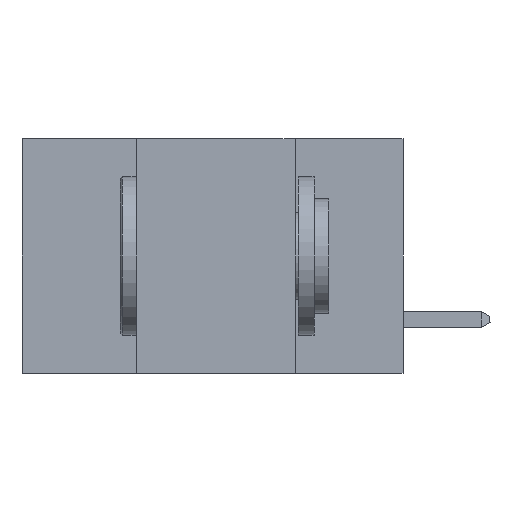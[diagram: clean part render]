
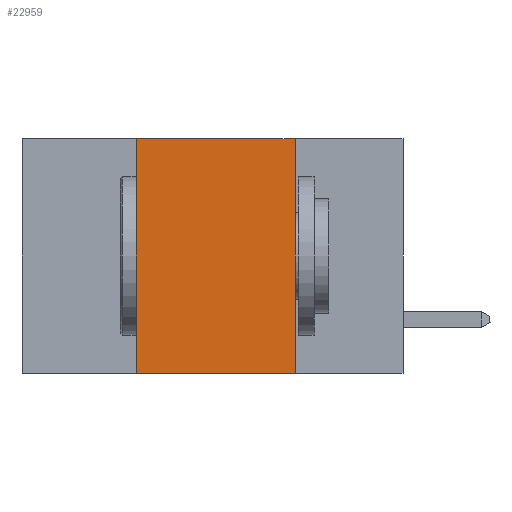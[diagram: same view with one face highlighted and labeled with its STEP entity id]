
A CAD part, left-side view. The second image highlights one B-rep face of the part: STEP entity #22959.
In plain terms, the highlighted planar face has unit normal (-1, 0, 0).
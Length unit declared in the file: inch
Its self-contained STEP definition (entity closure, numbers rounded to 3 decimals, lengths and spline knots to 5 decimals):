
#614 = VERTEX_POINT ( 'NONE', #19256 ) ;
#2746 = VECTOR ( 'NONE', #14389, 39.37008 ) ;
#2916 = DIRECTION ( 'NONE',  ( 0., 0., -1. ) ) ;
#3272 = CARTESIAN_POINT ( 'NONE',  ( 0., 0.6, -0.37 ) ) ;
#3844 = CARTESIAN_POINT ( 'NONE',  ( 0., 0.6, 0. ) ) ;
#3864 = CARTESIAN_POINT ( 'NONE',  ( 0., 0.17, 0. ) ) ;
#3929 = CARTESIAN_POINT ( 'NONE',  ( 0., 0.17, -0.37 ) ) ;
#5118 = VERTEX_POINT ( 'NONE', #3929 ) ;
#6164 = ORIENTED_EDGE ( 'NONE', *, *, #10696, .F. ) ;
#6297 = EDGE_LOOP ( 'NONE', ( #10286, #9710, #6164, #18606 ) ) ;
#6323 = VERTEX_POINT ( 'NONE', #9676 ) ;
#7345 = VECTOR ( 'NONE', #12236, 39.37008 ) ;
#7676 = VECTOR ( 'NONE', #19386, 39.37008 ) ;
#7748 = EDGE_CURVE ( 'NONE', #614, #5118, #13278, .T. ) ;
#8371 = CARTESIAN_POINT ( 'NONE',  ( 0., 0.6, 0. ) ) ;
#8465 = LINE ( 'NONE', #15221, #11813 ) ;
#9676 = CARTESIAN_POINT ( 'NONE',  ( 0., 0.42, 0. ) ) ;
#9710 = ORIENTED_EDGE ( 'NONE', *, *, #17797, .F. ) ;
#10286 = ORIENTED_EDGE ( 'NONE', *, *, #10840, .F. ) ;
#10696 = EDGE_CURVE ( 'NONE', #614, #6323, #10721, .T. ) ;
#10721 = LINE ( 'NONE', #15592, #7345 ) ;
#10840 = EDGE_CURVE ( 'NONE', #22556, #5118, #8465, .T. ) ;
#11813 = VECTOR ( 'NONE', #2916, 39.37008 ) ;
#12236 = DIRECTION ( 'NONE',  ( 0., 0., 1. ) ) ;
#12377 = PLANE ( 'NONE',  #13827 ) ;
#13278 = LINE ( 'NONE', #3272, #7676 ) ;
#13827 = AXIS2_PLACEMENT_3D ( 'NONE', #8371, #17353, #22699 ) ;
#14258 = LINE ( 'NONE', #3844, #2746 ) ;
#14389 = DIRECTION ( 'NONE',  ( 0., -1., 0. ) ) ;
#15221 = CARTESIAN_POINT ( 'NONE',  ( 0., 0.17, 0. ) ) ;
#15592 = CARTESIAN_POINT ( 'NONE',  ( 0., 0.42, 0. ) ) ;
#17353 = DIRECTION ( 'NONE',  ( 1., 0., 0. ) ) ;
#17797 = EDGE_CURVE ( 'NONE', #6323, #22556, #14258, .T. ) ;
#17884 = FACE_OUTER_BOUND ( 'NONE', #6297, .T. ) ;
#18606 = ORIENTED_EDGE ( 'NONE', *, *, #7748, .T. ) ;
#19256 = CARTESIAN_POINT ( 'NONE',  ( 0., 0.42, -0.37 ) ) ;
#19386 = DIRECTION ( 'NONE',  ( 0., -1., 0. ) ) ;
#22556 = VERTEX_POINT ( 'NONE', #3864 ) ;
#22699 = DIRECTION ( 'NONE',  ( 0., 0., -1. ) ) ;
#22959 = ADVANCED_FACE ( 'NONE', ( #17884 ), #12377, .F. ) ;
